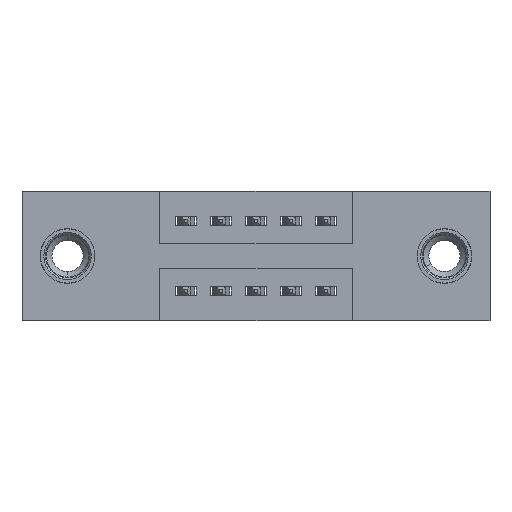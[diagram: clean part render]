
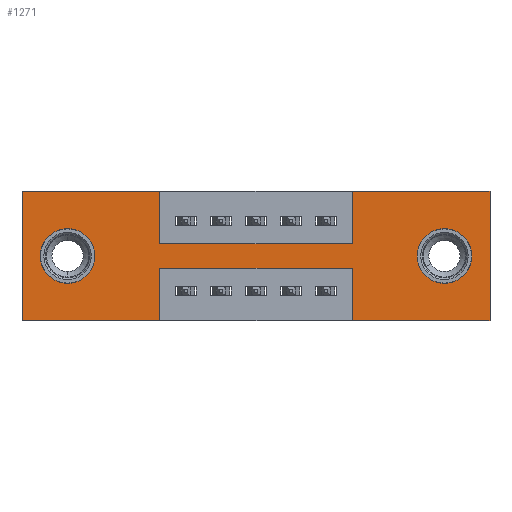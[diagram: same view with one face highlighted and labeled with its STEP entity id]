
A CAD part, front view. The second image highlights one B-rep face of the part: STEP entity #1271.
In plain terms, the highlighted planar face has unit normal (0, -1, 0).
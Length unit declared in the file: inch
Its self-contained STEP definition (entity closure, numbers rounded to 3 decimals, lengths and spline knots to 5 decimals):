
#120 = VERTEX_POINT ( 'NONE', #3722 ) ;
#210 = CIRCLE ( 'NONE', #8091, 0.078 ) ;
#268 = LINE ( 'NONE', #7173, #2143 ) ;
#314 = VECTOR ( 'NONE', #9098, 39.37008 ) ;
#365 = VECTOR ( 'NONE', #5315, 39.37008 ) ;
#644 = CARTESIAN_POINT ( 'NONE',  ( 0., 0., -0.37 ) ) ;
#778 = EDGE_CURVE ( 'NONE', #2192, #7449, #8008, .T. ) ;
#816 = VERTEX_POINT ( 'NONE', #7539 ) ;
#846 = DIRECTION ( 'NONE',  ( 0., 0., -1. ) ) ;
#861 = DIRECTION ( 'NONE',  ( 0., 1., 0. ) ) ;
#903 = EDGE_LOOP ( 'NONE', ( #4580, #1842 ) ) ;
#950 = VERTEX_POINT ( 'NONE', #4066 ) ;
#955 = ORIENTED_EDGE ( 'NONE', *, *, #6652, .F. ) ;
#970 = EDGE_CURVE ( 'NONE', #6958, #950, #6495, .T. ) ;
#984 = CARTESIAN_POINT ( 'NONE',  ( 0.13, 0., -0.185 ) ) ;
#1062 = CARTESIAN_POINT ( 'NONE',  ( 1.205, 0., -0.185 ) ) ;
#1271 = ADVANCED_FACE ( 'NONE', ( #2045, #4318, #6615 ), #3019, .T. ) ;
#1339 = CARTESIAN_POINT ( 'NONE',  ( 0.9425, 0., -0.37 ) ) ;
#1721 = CARTESIAN_POINT ( 'NONE',  ( 0.13, 0., -0.107 ) ) ;
#1803 = DIRECTION ( 'NONE',  ( 0., 0., 1. ) ) ;
#1842 = ORIENTED_EDGE ( 'NONE', *, *, #1941, .T. ) ;
#1941 = EDGE_CURVE ( 'NONE', #4701, #2200, #2150, .T. ) ;
#1974 = DIRECTION ( 'NONE',  ( 1., 0., 0. ) ) ;
#2020 = LINE ( 'NONE', #5387, #2256 ) ;
#2045 = FACE_BOUND ( 'NONE', #903, .T. ) ;
#2086 = ORIENTED_EDGE ( 'NONE', *, *, #5079, .F. ) ;
#2143 = VECTOR ( 'NONE', #7208, 39.37008 ) ;
#2150 = CIRCLE ( 'NONE', #6374, 0.078 ) ;
#2192 = VERTEX_POINT ( 'NONE', #8641 ) ;
#2200 = VERTEX_POINT ( 'NONE', #8582 ) ;
#2224 = VECTOR ( 'NONE', #7768, 39.37008 ) ;
#2256 = VECTOR ( 'NONE', #5763, 39.37008 ) ;
#2291 = VECTOR ( 'NONE', #10111, 39.37008 ) ;
#2369 = EDGE_CURVE ( 'NONE', #7449, #5910, #268, .T. ) ;
#2374 = VERTEX_POINT ( 'NONE', #7081 ) ;
#2442 = EDGE_CURVE ( 'NONE', #2995, #6958, #7601, .T. ) ;
#2471 = LINE ( 'NONE', #8475, #365 ) ;
#2484 = CARTESIAN_POINT ( 'NONE',  ( 1.335, 0., -0.37 ) ) ;
#2625 = EDGE_CURVE ( 'NONE', #5243, #2995, #2020, .T. ) ;
#2627 = CARTESIAN_POINT ( 'NONE',  ( 0., 0., 0. ) ) ;
#2646 = VECTOR ( 'NONE', #7761, 39.37008 ) ;
#2877 = EDGE_CURVE ( 'NONE', #5910, #7960, #3442, .T. ) ;
#2995 = VERTEX_POINT ( 'NONE', #2484 ) ;
#3019 = PLANE ( 'NONE',  #3670 ) ;
#3147 = ORIENTED_EDGE ( 'NONE', *, *, #7893, .F. ) ;
#3195 = CARTESIAN_POINT ( 'NONE',  ( 0.9425, 0., 0. ) ) ;
#3232 = DIRECTION ( 'NONE',  ( 0., 0., 1. ) ) ;
#3367 = DIRECTION ( 'NONE',  ( 0., 1., 0. ) ) ;
#3442 = LINE ( 'NONE', #3195, #7347 ) ;
#3451 = VERTEX_POINT ( 'NONE', #1721 ) ;
#3509 = CARTESIAN_POINT ( 'NONE',  ( 0., 0., 0. ) ) ;
#3560 = EDGE_CURVE ( 'NONE', #7441, #120, #9276, .T. ) ;
#3580 = CARTESIAN_POINT ( 'NONE',  ( 0.9425, 0., 0. ) ) ;
#3670 = AXIS2_PLACEMENT_3D ( 'NONE', #8879, #4226, #6050 ) ;
#3722 = CARTESIAN_POINT ( 'NONE',  ( 0., 0., 0. ) ) ;
#3736 = CARTESIAN_POINT ( 'NONE',  ( 0., 0., -0.37 ) ) ;
#3804 = CIRCLE ( 'NONE', #7097, 0.078 ) ;
#3847 = VECTOR ( 'NONE', #1974, 39.37008 ) ;
#3931 = DIRECTION ( 'NONE',  ( 0., 1., 0. ) ) ;
#4066 = CARTESIAN_POINT ( 'NONE',  ( 0.9425, 0., -0.22 ) ) ;
#4130 = ORIENTED_EDGE ( 'NONE', *, *, #3560, .F. ) ;
#4226 = DIRECTION ( 'NONE',  ( 0., -1., 0. ) ) ;
#4260 = LINE ( 'NONE', #9320, #2224 ) ;
#4318 = FACE_BOUND ( 'NONE', #5983, .T. ) ;
#4580 = ORIENTED_EDGE ( 'NONE', *, *, #5732, .T. ) ;
#4701 = VERTEX_POINT ( 'NONE', #7938 ) ;
#4987 = DIRECTION ( 'NONE',  ( 0., 0., 1. ) ) ;
#5079 = EDGE_CURVE ( 'NONE', #120, #2192, #4260, .T. ) ;
#5119 = VECTOR ( 'NONE', #4987, 39.37008 ) ;
#5243 = VERTEX_POINT ( 'NONE', #5642 ) ;
#5254 = AXIS2_PLACEMENT_3D ( 'NONE', #984, #6398, #1803 ) ;
#5315 = DIRECTION ( 'NONE',  ( -1., 0., 0. ) ) ;
#5387 = CARTESIAN_POINT ( 'NONE',  ( 1.335, 0., 0. ) ) ;
#5492 = VECTOR ( 'NONE', #6569, 39.37008 ) ;
#5574 = EDGE_CURVE ( 'NONE', #816, #7441, #5797, .T. ) ;
#5642 = CARTESIAN_POINT ( 'NONE',  ( 1.335, 0., 0. ) ) ;
#5678 = ORIENTED_EDGE ( 'NONE', *, *, #2877, .F. ) ;
#5732 = EDGE_CURVE ( 'NONE', #2200, #4701, #210, .T. ) ;
#5763 = DIRECTION ( 'NONE',  ( 0., 0., -1. ) ) ;
#5797 = LINE ( 'NONE', #3736, #7912 ) ;
#5910 = VERTEX_POINT ( 'NONE', #8066 ) ;
#5923 = ORIENTED_EDGE ( 'NONE', *, *, #2369, .F. ) ;
#5983 = EDGE_LOOP ( 'NONE', ( #8303, #8792 ) ) ;
#6035 = ORIENTED_EDGE ( 'NONE', *, *, #970, .F. ) ;
#6050 = DIRECTION ( 'NONE',  ( 0., 0., -1. ) ) ;
#6374 = AXIS2_PLACEMENT_3D ( 'NONE', #1062, #861, #846 ) ;
#6398 = DIRECTION ( 'NONE',  ( 0., 1., 0. ) ) ;
#6495 = LINE ( 'NONE', #1339, #2646 ) ;
#6569 = DIRECTION ( 'NONE',  ( -1., 0., 0. ) ) ;
#6590 = CARTESIAN_POINT ( 'NONE',  ( 0.13, 0., -0.263 ) ) ;
#6603 = CARTESIAN_POINT ( 'NONE',  ( 0.3925, 0., 0. ) ) ;
#6615 = FACE_OUTER_BOUND ( 'NONE', #9116, .T. ) ;
#6652 = EDGE_CURVE ( 'NONE', #2374, #816, #8662, .T. ) ;
#6771 = CARTESIAN_POINT ( 'NONE',  ( 0., 0., -0.37 ) ) ;
#6802 = DIRECTION ( 'NONE',  ( -1., 0., 0. ) ) ;
#6868 = CARTESIAN_POINT ( 'NONE',  ( 0.3925, 0., -0.15 ) ) ;
#6958 = VERTEX_POINT ( 'NONE', #7919 ) ;
#7026 = ORIENTED_EDGE ( 'NONE', *, *, #2625, .F. ) ;
#7081 = CARTESIAN_POINT ( 'NONE',  ( 0.3925, 0., -0.22 ) ) ;
#7097 = AXIS2_PLACEMENT_3D ( 'NONE', #8049, #3367, #8848 ) ;
#7173 = CARTESIAN_POINT ( 'NONE',  ( 0.3925, 0., -0.15 ) ) ;
#7208 = DIRECTION ( 'NONE',  ( 1., 0., 0. ) ) ;
#7234 = VERTEX_POINT ( 'NONE', #6590 ) ;
#7347 = VECTOR ( 'NONE', #3232, 39.37008 ) ;
#7441 = VERTEX_POINT ( 'NONE', #644 ) ;
#7449 = VERTEX_POINT ( 'NONE', #6868 ) ;
#7539 = CARTESIAN_POINT ( 'NONE',  ( 0.3925, 0., -0.37 ) ) ;
#7601 = LINE ( 'NONE', #6771, #5492 ) ;
#7761 = DIRECTION ( 'NONE',  ( 0., 0., 1. ) ) ;
#7768 = DIRECTION ( 'NONE',  ( 1., 0., 0. ) ) ;
#7893 = EDGE_CURVE ( 'NONE', #7960, #5243, #10060, .T. ) ;
#7912 = VECTOR ( 'NONE', #6802, 39.37008 ) ;
#7919 = CARTESIAN_POINT ( 'NONE',  ( 0.9425, 0., -0.37 ) ) ;
#7938 = CARTESIAN_POINT ( 'NONE',  ( 1.205, 0., -0.263 ) ) ;
#7960 = VERTEX_POINT ( 'NONE', #3580 ) ;
#7984 = CIRCLE ( 'NONE', #5254, 0.078 ) ;
#8008 = LINE ( 'NONE', #6603, #2291 ) ;
#8043 = ORIENTED_EDGE ( 'NONE', *, *, #778, .F. ) ;
#8049 = CARTESIAN_POINT ( 'NONE',  ( 0.13, 0., -0.185 ) ) ;
#8066 = CARTESIAN_POINT ( 'NONE',  ( 0.9425, 0., -0.15 ) ) ;
#8091 = AXIS2_PLACEMENT_3D ( 'NONE', #8638, #3931, #9370 ) ;
#8303 = ORIENTED_EDGE ( 'NONE', *, *, #8376, .T. ) ;
#8311 = ORIENTED_EDGE ( 'NONE', *, *, #5574, .F. ) ;
#8376 = EDGE_CURVE ( 'NONE', #3451, #7234, #7984, .T. ) ;
#8425 = ORIENTED_EDGE ( 'NONE', *, *, #2442, .F. ) ;
#8475 = CARTESIAN_POINT ( 'NONE',  ( 0.3925, 0., -0.22 ) ) ;
#8582 = CARTESIAN_POINT ( 'NONE',  ( 1.205, 0., -0.107 ) ) ;
#8638 = CARTESIAN_POINT ( 'NONE',  ( 1.205, 0., -0.185 ) ) ;
#8641 = CARTESIAN_POINT ( 'NONE',  ( 0.3925, 0., 0. ) ) ;
#8662 = LINE ( 'NONE', #9002, #314 ) ;
#8792 = ORIENTED_EDGE ( 'NONE', *, *, #9656, .T. ) ;
#8848 = DIRECTION ( 'NONE',  ( 0., 0., 1. ) ) ;
#8879 = CARTESIAN_POINT ( 'NONE',  ( 0., 0., -0.37 ) ) ;
#9002 = CARTESIAN_POINT ( 'NONE',  ( 0.3925, 0., -0.37 ) ) ;
#9098 = DIRECTION ( 'NONE',  ( 0., 0., -1. ) ) ;
#9116 = EDGE_LOOP ( 'NONE', ( #955, #9240, #6035, #8425, #7026, #3147, #5678, #5923, #8043, #2086, #4130, #8311 ) ) ;
#9240 = ORIENTED_EDGE ( 'NONE', *, *, #9993, .F. ) ;
#9276 = LINE ( 'NONE', #2627, #5119 ) ;
#9320 = CARTESIAN_POINT ( 'NONE',  ( 0., 0., 0. ) ) ;
#9370 = DIRECTION ( 'NONE',  ( 0., 0., -1. ) ) ;
#9656 = EDGE_CURVE ( 'NONE', #7234, #3451, #3804, .T. ) ;
#9993 = EDGE_CURVE ( 'NONE', #950, #2374, #2471, .T. ) ;
#10060 = LINE ( 'NONE', #3509, #3847 ) ;
#10111 = DIRECTION ( 'NONE',  ( 0., 0., -1. ) ) ;
